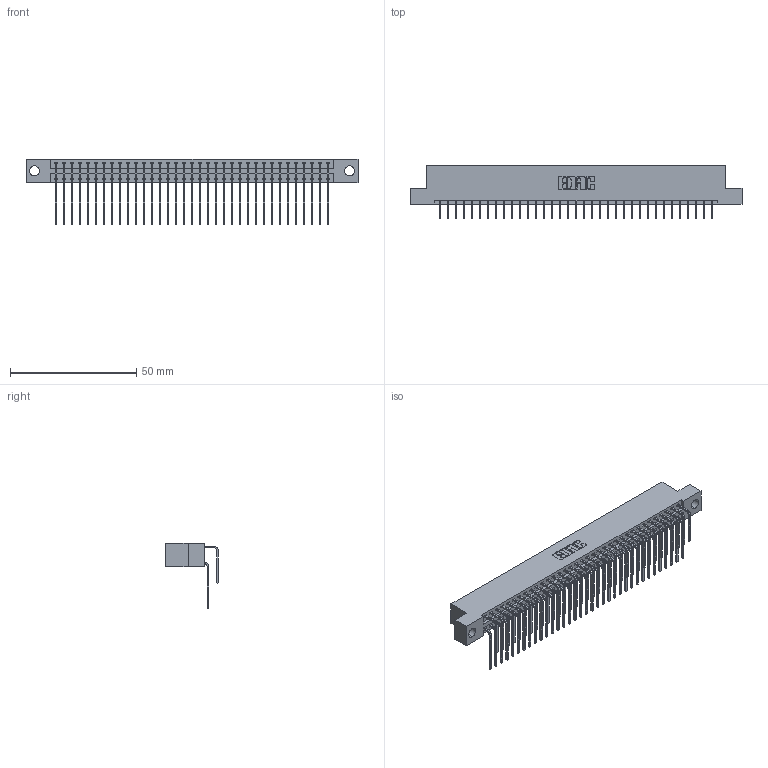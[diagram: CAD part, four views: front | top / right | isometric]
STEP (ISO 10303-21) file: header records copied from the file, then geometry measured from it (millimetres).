
FILE_DESCRIPTION (( 'STEP AP203' ), '1' );
FILE_NAME ('346-070-559-204.STEP', '2018-08-28T23:57:18', ( '' ), ( '' ), 'SwSTEP 2.0', 'SolidWorks 2016', '' );
FILE_SCHEMA (( 'CONFIG_CONTROL_DESIGN' ));
Length unit declared in the file: inch
Products named in the file (4): 346 Part_Flush Mounting Lugs - 0.156 Dia-TH; 345-292-001_558 559 Tail - 1; 345-292-001_559 Tail - 2; 346-070-559-204
Assembly tree (71 placements, depth 2):
  346-070-559-204
    346 Part_Flush Mounting Lugs - 0.156 Dia-TH
    345-292-001_558 559 Tail - 1  x35
    345-292-001_559 Tail - 2  x35
Bounding box: 131.7 x 20.89 x 26.16 mm (x, y, z)
Volume: 13103.9 mm3; surface area: 19652.7 mm2
Topology: 71 solids, 71 shells, 3902 faces, 11599 edges, 7638 vertices
Faces by surface type: plane 2666, cylinder 1236
Entity records: 25571 total; most frequent: CARTESIAN_POINT 4275, ORIENTED_EDGE 4158, DIRECTION 3791, EDGE_CURVE 2079, VECTOR 1767, LINE 1767, VERTEX_POINT 1382, AXIS2_PLACEMENT_3D 1012
